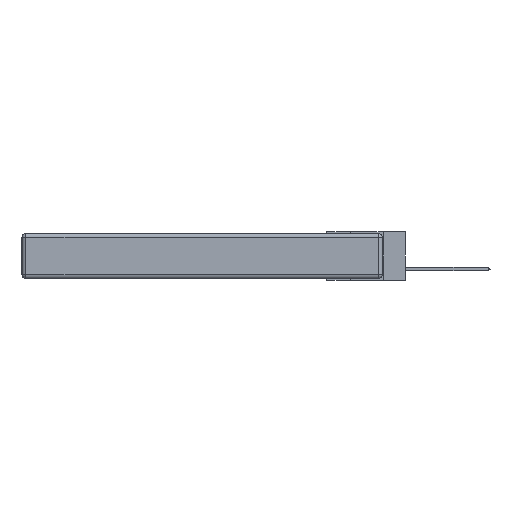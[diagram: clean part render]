
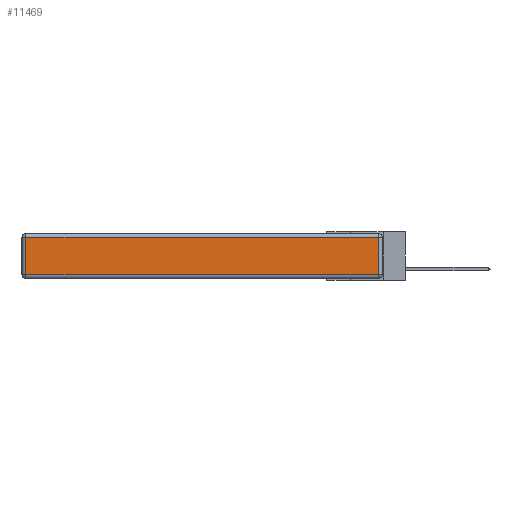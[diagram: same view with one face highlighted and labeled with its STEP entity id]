
A CAD part, left-side view. The second image highlights one B-rep face of the part: STEP entity #11469.
In plain terms, the highlighted planar face has unit normal (-1, 0, 0).
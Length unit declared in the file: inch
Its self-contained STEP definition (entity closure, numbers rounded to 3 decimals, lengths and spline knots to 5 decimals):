
#849 = DIRECTION ( 'NONE',  ( -1., 0., 0. ) ) ;
#2015 = LINE ( 'NONE', #12985, #16411 ) ;
#4133 = CARTESIAN_POINT ( 'NONE',  ( 0., 2.72, -0.343 ) ) ;
#4463 = LINE ( 'NONE', #9488, #18814 ) ;
#5639 = FACE_OUTER_BOUND ( 'NONE', #11698, .T. ) ;
#6003 = ORIENTED_EDGE ( 'NONE', *, *, #12785, .T. ) ;
#6351 = DIRECTION ( 'NONE',  ( 0., 0., 1. ) ) ;
#7075 = LINE ( 'NONE', #20143, #10599 ) ;
#8029 = DIRECTION ( 'NONE',  ( 0., 0., 1. ) ) ;
#8740 = VERTEX_POINT ( 'NONE', #12706 ) ;
#9230 = CARTESIAN_POINT ( 'NONE',  ( 0., 0.03, -0.03 ) ) ;
#9488 = CARTESIAN_POINT ( 'NONE',  ( 0., 0.03, -0.343 ) ) ;
#9560 = DIRECTION ( 'NONE',  ( 0., 0., -1. ) ) ;
#9757 = CARTESIAN_POINT ( 'NONE',  ( 0., 0., -0.343 ) ) ;
#10599 = VECTOR ( 'NONE', #18548, 39.37008 ) ;
#10863 = EDGE_CURVE ( 'NONE', #8740, #18117, #21382, .T. ) ;
#11469 = ADVANCED_FACE ( 'NONE', ( #5639 ), #19860, .T. ) ;
#11698 = EDGE_LOOP ( 'NONE', ( #6003, #16528, #19709, #14792 ) ) ;
#11908 = VERTEX_POINT ( 'NONE', #9230 ) ;
#12338 = VERTEX_POINT ( 'NONE', #13007 ) ;
#12706 = CARTESIAN_POINT ( 'NONE',  ( 0., 2.72, -0.03 ) ) ;
#12785 = EDGE_CURVE ( 'NONE', #18117, #12338, #2015, .T. ) ;
#12985 = CARTESIAN_POINT ( 'NONE',  ( 0., 0., -0.313 ) ) ;
#13007 = CARTESIAN_POINT ( 'NONE',  ( 0., 0.03, -0.313 ) ) ;
#13757 = VECTOR ( 'NONE', #9560, 39.37008 ) ;
#14792 = ORIENTED_EDGE ( 'NONE', *, *, #10863, .T. ) ;
#14795 = CARTESIAN_POINT ( 'NONE',  ( 0., 2.72, -0.313 ) ) ;
#16411 = VECTOR ( 'NONE', #18297, 39.37008 ) ;
#16528 = ORIENTED_EDGE ( 'NONE', *, *, #19741, .T. ) ;
#18117 = VERTEX_POINT ( 'NONE', #14795 ) ;
#18297 = DIRECTION ( 'NONE',  ( 0., -1., 0. ) ) ;
#18503 = AXIS2_PLACEMENT_3D ( 'NONE', #9757, #849, #6351 ) ;
#18548 = DIRECTION ( 'NONE',  ( 0., 1., 0. ) ) ;
#18814 = VECTOR ( 'NONE', #8029, 39.37008 ) ;
#19709 = ORIENTED_EDGE ( 'NONE', *, *, #22360, .T. ) ;
#19741 = EDGE_CURVE ( 'NONE', #12338, #11908, #4463, .T. ) ;
#19860 = PLANE ( 'NONE',  #18503 ) ;
#20143 = CARTESIAN_POINT ( 'NONE',  ( 0., 2.75, -0.03 ) ) ;
#21382 = LINE ( 'NONE', #4133, #13757 ) ;
#22360 = EDGE_CURVE ( 'NONE', #11908, #8740, #7075, .T. ) ;
